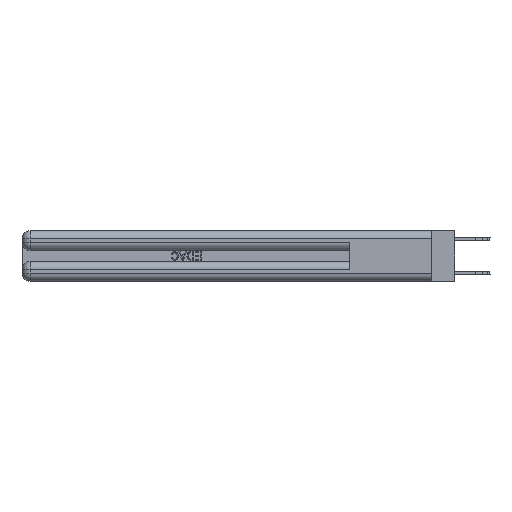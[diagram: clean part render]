
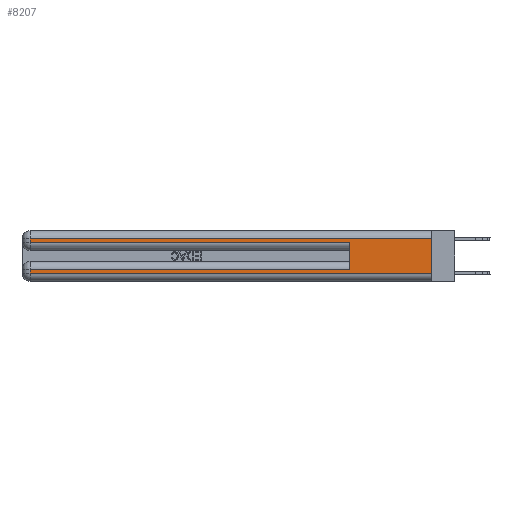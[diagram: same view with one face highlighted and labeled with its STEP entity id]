
A CAD part, left-side view. The second image highlights one B-rep face of the part: STEP entity #8207.
In plain terms, the highlighted planar face has unit normal (-1, 0, 0).
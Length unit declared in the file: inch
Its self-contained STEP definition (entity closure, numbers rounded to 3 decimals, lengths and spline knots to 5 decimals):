
#182 = ORIENTED_EDGE ( 'NONE', *, *, #15009, .T. ) ;
#215 = CARTESIAN_POINT ( 'NONE',  ( 0., 2.94, 0.31 ) ) ;
#1104 = ORIENTED_EDGE ( 'NONE', *, *, #9127, .T. ) ;
#2242 = DIRECTION ( 'NONE',  ( 0., 0., -1. ) ) ;
#2381 = DIRECTION ( 'NONE',  ( 1., 0., 0. ) ) ;
#2449 = CARTESIAN_POINT ( 'NONE',  ( 0., 0., 0.31 ) ) ;
#2599 = VECTOR ( 'NONE', #20231, 39.37008 ) ;
#2866 = LINE ( 'NONE', #11758, #24665 ) ;
#3208 = EDGE_CURVE ( 'NONE', #24719, #21589, #15312, .T. ) ;
#3784 = EDGE_CURVE ( 'NONE', #24719, #25108, #15705, .T. ) ;
#3939 = VECTOR ( 'NONE', #4207, 39.37008 ) ;
#4207 = DIRECTION ( 'NONE',  ( 0., 0., -1. ) ) ;
#4473 = AXIS2_PLACEMENT_3D ( 'NONE', #15525, #2381, #2242 ) ;
#4682 = ORIENTED_EDGE ( 'NONE', *, *, #15097, .T. ) ;
#5182 = EDGE_LOOP ( 'NONE', ( #18885, #6058, #26376, #9988, #9468, #182, #1104, #4682 ) ) ;
#5560 = VERTEX_POINT ( 'NONE', #21222 ) ;
#6058 = ORIENTED_EDGE ( 'NONE', *, *, #3784, .T. ) ;
#6220 = DIRECTION ( 'NONE',  ( 0., -1., 0. ) ) ;
#6752 = CARTESIAN_POINT ( 'NONE',  ( 0., 0.6, 0.145 ) ) ;
#7199 = CARTESIAN_POINT ( 'NONE',  ( 0., 0., 0.31 ) ) ;
#7946 = EDGE_CURVE ( 'NONE', #25108, #9312, #18642, .T. ) ;
#8069 = CARTESIAN_POINT ( 'NONE',  ( 0., 2.94, 0.285 ) ) ;
#8186 = EDGE_CURVE ( 'NONE', #28402, #14556, #21979, .T. ) ;
#8207 = ADVANCED_FACE ( 'NONE', ( #13035 ), #8927, .F. ) ;
#8243 = VECTOR ( 'NONE', #6220, 39.37008 ) ;
#8259 = LINE ( 'NONE', #28365, #8243 ) ;
#8927 = PLANE ( 'NONE',  #4473 ) ;
#9127 = EDGE_CURVE ( 'NONE', #28181, #5560, #2866, .T. ) ;
#9312 = VERTEX_POINT ( 'NONE', #8069 ) ;
#9403 = DIRECTION ( 'NONE',  ( 0., 0., -1. ) ) ;
#9468 = ORIENTED_EDGE ( 'NONE', *, *, #8186, .F. ) ;
#9988 = ORIENTED_EDGE ( 'NONE', *, *, #23537, .T. ) ;
#11435 = DIRECTION ( 'NONE',  ( 0., 0., 1. ) ) ;
#11634 = CARTESIAN_POINT ( 'NONE',  ( 0., 0.6, 0.285 ) ) ;
#11652 = CARTESIAN_POINT ( 'NONE',  ( 0., 0.6, 0.085 ) ) ;
#11758 = CARTESIAN_POINT ( 'NONE',  ( 0., 2.94, 0.37 ) ) ;
#13035 = FACE_OUTER_BOUND ( 'NONE', #5182, .T. ) ;
#13072 = CARTESIAN_POINT ( 'NONE',  ( 0., 0., 0.06 ) ) ;
#13293 = VECTOR ( 'NONE', #9403, 39.37008 ) ;
#14233 = CARTESIAN_POINT ( 'NONE',  ( 0., 2.94, 0.37 ) ) ;
#14504 = LINE ( 'NONE', #19044, #20523 ) ;
#14556 = VERTEX_POINT ( 'NONE', #11634 ) ;
#15009 = EDGE_CURVE ( 'NONE', #28402, #28181, #28014, .T. ) ;
#15097 = EDGE_CURVE ( 'NONE', #5560, #21589, #14504, .T. ) ;
#15312 = LINE ( 'NONE', #26196, #3939 ) ;
#15525 = CARTESIAN_POINT ( 'NONE',  ( 0., 0., 0.37 ) ) ;
#15705 = LINE ( 'NONE', #7199, #2599 ) ;
#16313 = VECTOR ( 'NONE', #23397, 39.37008 ) ;
#17129 = CARTESIAN_POINT ( 'NONE',  ( 0., 0., 0.085 ) ) ;
#18642 = LINE ( 'NONE', #14233, #13293 ) ;
#18646 = DIRECTION ( 'NONE',  ( 0., 0., -1. ) ) ;
#18885 = ORIENTED_EDGE ( 'NONE', *, *, #3208, .F. ) ;
#19044 = CARTESIAN_POINT ( 'NONE',  ( 0., 0., 0.06 ) ) ;
#20144 = CARTESIAN_POINT ( 'NONE',  ( 0., 2.94, 0.085 ) ) ;
#20231 = DIRECTION ( 'NONE',  ( 0., 1., 0. ) ) ;
#20523 = VECTOR ( 'NONE', #25264, 39.37008 ) ;
#21222 = CARTESIAN_POINT ( 'NONE',  ( 0., 2.94, 0.06 ) ) ;
#21589 = VERTEX_POINT ( 'NONE', #13072 ) ;
#21979 = LINE ( 'NONE', #6752, #26004 ) ;
#23397 = DIRECTION ( 'NONE',  ( 0., 1., 0. ) ) ;
#23537 = EDGE_CURVE ( 'NONE', #9312, #14556, #8259, .T. ) ;
#24665 = VECTOR ( 'NONE', #18646, 39.37008 ) ;
#24719 = VERTEX_POINT ( 'NONE', #2449 ) ;
#25108 = VERTEX_POINT ( 'NONE', #215 ) ;
#25264 = DIRECTION ( 'NONE',  ( 0., -1., 0. ) ) ;
#26004 = VECTOR ( 'NONE', #11435, 39.37008 ) ;
#26196 = CARTESIAN_POINT ( 'NONE',  ( 0., 0., 0.37 ) ) ;
#26376 = ORIENTED_EDGE ( 'NONE', *, *, #7946, .T. ) ;
#28014 = LINE ( 'NONE', #17129, #16313 ) ;
#28181 = VERTEX_POINT ( 'NONE', #20144 ) ;
#28365 = CARTESIAN_POINT ( 'NONE',  ( 0., 0., 0.285 ) ) ;
#28402 = VERTEX_POINT ( 'NONE', #11652 ) ;
